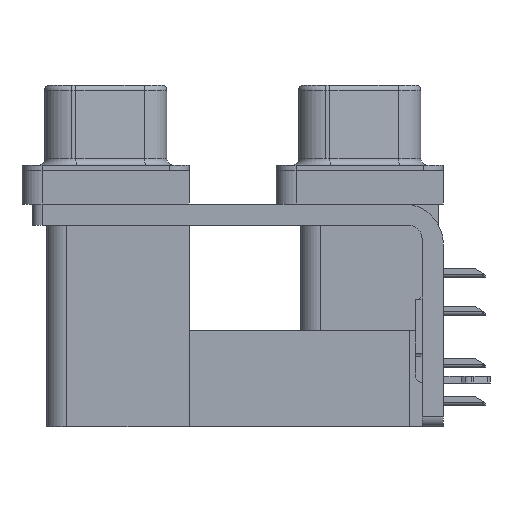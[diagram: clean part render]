
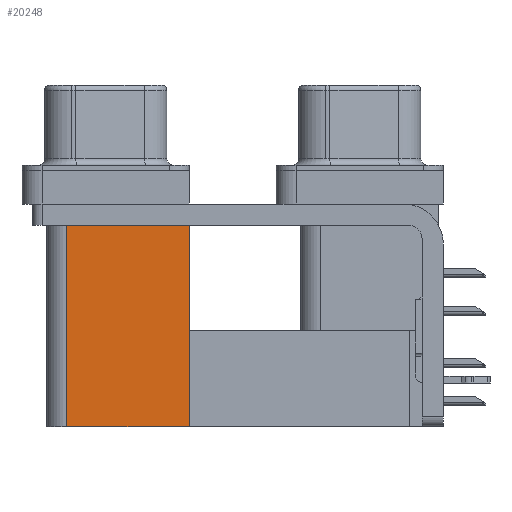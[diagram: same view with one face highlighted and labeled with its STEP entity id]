
A CAD part, left-side view. The second image highlights one B-rep face of the part: STEP entity #20248.
In plain terms, the highlighted planar face has unit normal (-1, 0, 0).
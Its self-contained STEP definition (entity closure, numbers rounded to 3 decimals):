
#853 = LINE ( 'NONE', #32183, #2478 ) ;
#2478 = VECTOR ( 'NONE', #11134, 1000. ) ;
#3298 = ORIENTED_EDGE ( 'NONE', *, *, #20172, .F. ) ;
#3511 = CARTESIAN_POINT ( 'NONE',  ( 3.765, 12.775, -19.2 ) ) ;
#5202 = CARTESIAN_POINT ( 'NONE',  ( 3.765, 12.775, -19.2 ) ) ;
#5216 = ORIENTED_EDGE ( 'NONE', *, *, #28677, .T. ) ;
#5866 = LINE ( 'NONE', #3511, #30966 ) ;
#6102 = LINE ( 'NONE', #32058, #29218 ) ;
#7072 = VERTEX_POINT ( 'NONE', #7908 ) ;
#7908 = CARTESIAN_POINT ( 'NONE',  ( 3.765, 21.975, -2.5 ) ) ;
#8620 = EDGE_LOOP ( 'NONE', ( #5216, #30721, #3298, #17286 ) ) ;
#8707 = FACE_OUTER_BOUND ( 'NONE', #8620, .T. ) ;
#10034 = PLANE ( 'NONE',  #14306 ) ;
#10708 = CARTESIAN_POINT ( 'NONE',  ( 3.765, 21.975, -19.2 ) ) ;
#11134 = DIRECTION ( 'NONE',  ( 0., 0., 1. ) ) ;
#12255 = DIRECTION ( 'NONE',  ( 1., 0., 0. ) ) ;
#12399 = VERTEX_POINT ( 'NONE', #24051 ) ;
#13998 = EDGE_CURVE ( 'NONE', #17520, #7072, #853, .T. ) ;
#14306 = AXIS2_PLACEMENT_3D ( 'NONE', #16977, #12255, #24898 ) ;
#15319 = CARTESIAN_POINT ( 'NONE',  ( 3.765, 12.775, -19.2 ) ) ;
#15721 = EDGE_CURVE ( 'NONE', #30780, #12399, #18351, .T. ) ;
#16977 = CARTESIAN_POINT ( 'NONE',  ( 3.765, 12.775, -19.2 ) ) ;
#17286 = ORIENTED_EDGE ( 'NONE', *, *, #15721, .T. ) ;
#17520 = VERTEX_POINT ( 'NONE', #10708 ) ;
#18351 = LINE ( 'NONE', #5202, #26732 ) ;
#20172 = EDGE_CURVE ( 'NONE', #30780, #17520, #5866, .T. ) ;
#20248 = ADVANCED_FACE ( 'NONE', ( #8707 ), #10034, .F. ) ;
#24051 = CARTESIAN_POINT ( 'NONE',  ( 3.765, 12.775, -2.5 ) ) ;
#24149 = DIRECTION ( 'NONE',  ( 0., 1., 0. ) ) ;
#24898 = DIRECTION ( 'NONE',  ( 0., 1., 0. ) ) ;
#26592 = DIRECTION ( 'NONE',  ( 0., 1., 0. ) ) ;
#26732 = VECTOR ( 'NONE', #28636, 1000. ) ;
#28636 = DIRECTION ( 'NONE',  ( 0., 0., 1. ) ) ;
#28677 = EDGE_CURVE ( 'NONE', #12399, #7072, #6102, .T. ) ;
#29218 = VECTOR ( 'NONE', #24149, 1000. ) ;
#30721 = ORIENTED_EDGE ( 'NONE', *, *, #13998, .F. ) ;
#30780 = VERTEX_POINT ( 'NONE', #15319 ) ;
#30966 = VECTOR ( 'NONE', #26592, 1000. ) ;
#32058 = CARTESIAN_POINT ( 'NONE',  ( 3.765, 12.775, -2.5 ) ) ;
#32183 = CARTESIAN_POINT ( 'NONE',  ( 3.765, 21.975, -19.2 ) ) ;
